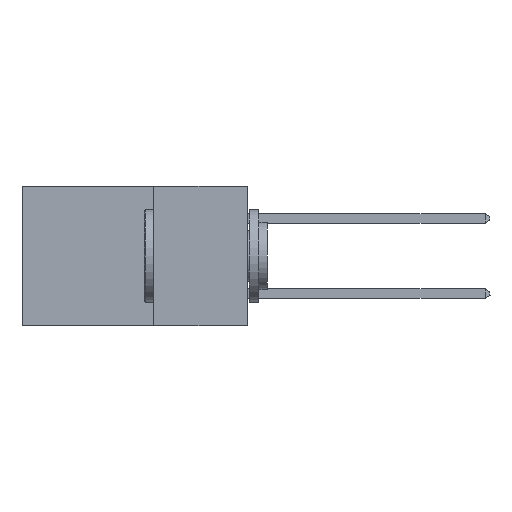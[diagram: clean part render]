
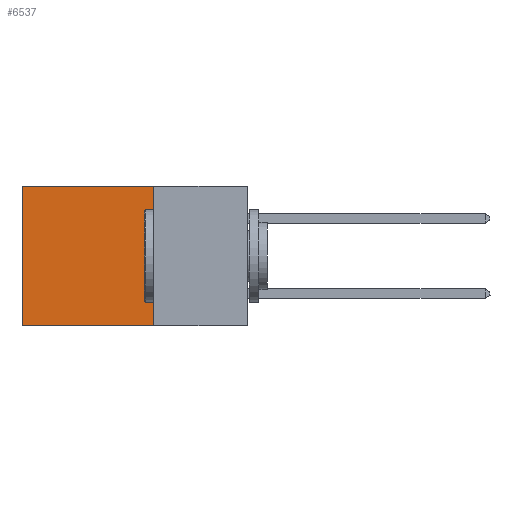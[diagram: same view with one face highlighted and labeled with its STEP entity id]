
A CAD part, left-side view. The second image highlights one B-rep face of the part: STEP entity #6537.
In plain terms, the highlighted planar face has unit normal (-1, 0, 0).
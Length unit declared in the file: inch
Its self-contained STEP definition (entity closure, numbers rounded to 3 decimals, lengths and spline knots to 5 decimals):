
#168 = AXIS2_PLACEMENT_3D ( 'NONE', #12115, #12182, #6692 ) ;
#2185 = CARTESIAN_POINT ( 'NONE',  ( 0.298, 0.25, -0.37 ) ) ;
#2479 = VERTEX_POINT ( 'NONE', #9520 ) ;
#2827 = CARTESIAN_POINT ( 'NONE',  ( 0.298, 0.6, 0. ) ) ;
#2900 = LINE ( 'NONE', #3617, #10000 ) ;
#3400 = VECTOR ( 'NONE', #11154, 39.37008 ) ;
#3617 = CARTESIAN_POINT ( 'NONE',  ( 0.298, 0.25, -0.37 ) ) ;
#4101 = VERTEX_POINT ( 'NONE', #17647 ) ;
#4161 = VERTEX_POINT ( 'NONE', #9085 ) ;
#4416 = ORIENTED_EDGE ( 'NONE', *, *, #5034, .F. ) ;
#4517 = DIRECTION ( 'NONE',  ( 0., 0., -1. ) ) ;
#4674 = ORIENTED_EDGE ( 'NONE', *, *, #16373, .T. ) ;
#4893 = ORIENTED_EDGE ( 'NONE', *, *, #8790, .F. ) ;
#5034 = EDGE_CURVE ( 'NONE', #17193, #4161, #2900, .T. ) ;
#5537 = FACE_OUTER_BOUND ( 'NONE', #14926, .T. ) ;
#6537 = ADVANCED_FACE ( 'NONE', ( #5537 ), #10818, .F. ) ;
#6692 = DIRECTION ( 'NONE',  ( 0., 0., -1. ) ) ;
#6835 = ORIENTED_EDGE ( 'NONE', *, *, #7887, .T. ) ;
#7757 = CARTESIAN_POINT ( 'NONE',  ( 0.298, 0.25, 0. ) ) ;
#7887 = EDGE_CURVE ( 'NONE', #2479, #4101, #12285, .T. ) ;
#8790 = EDGE_CURVE ( 'NONE', #2479, #17193, #12004, .T. ) ;
#9085 = CARTESIAN_POINT ( 'NONE',  ( 0.298, 0.6, -0.37 ) ) ;
#9520 = CARTESIAN_POINT ( 'NONE',  ( 0.298, 0.25, 0. ) ) ;
#10000 = VECTOR ( 'NONE', #10983, 39.37008 ) ;
#10818 = PLANE ( 'NONE',  #168 ) ;
#10983 = DIRECTION ( 'NONE',  ( 0., 1., 0. ) ) ;
#11154 = DIRECTION ( 'NONE',  ( 0., 1., 0. ) ) ;
#12004 = LINE ( 'NONE', #7757, #13345 ) ;
#12115 = CARTESIAN_POINT ( 'NONE',  ( 0.298, 0.25, 0. ) ) ;
#12182 = DIRECTION ( 'NONE',  ( 1., 0., 0. ) ) ;
#12285 = LINE ( 'NONE', #18252, #3400 ) ;
#13345 = VECTOR ( 'NONE', #13623, 39.37008 ) ;
#13379 = LINE ( 'NONE', #2827, #17642 ) ;
#13623 = DIRECTION ( 'NONE',  ( 0., 0., -1. ) ) ;
#14926 = EDGE_LOOP ( 'NONE', ( #4674, #4416, #4893, #6835 ) ) ;
#16373 = EDGE_CURVE ( 'NONE', #4101, #4161, #13379, .T. ) ;
#17193 = VERTEX_POINT ( 'NONE', #2185 ) ;
#17642 = VECTOR ( 'NONE', #4517, 39.37008 ) ;
#17647 = CARTESIAN_POINT ( 'NONE',  ( 0.298, 0.6, 0. ) ) ;
#18252 = CARTESIAN_POINT ( 'NONE',  ( 0.298, 0.25, 0. ) ) ;
